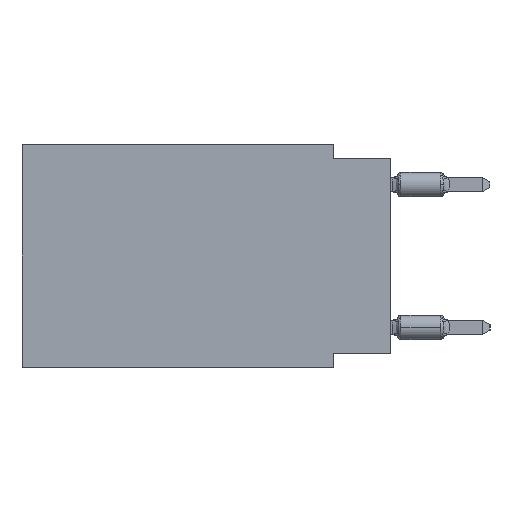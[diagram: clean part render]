
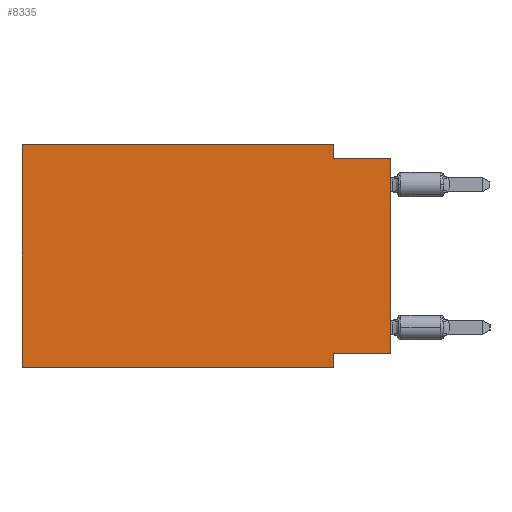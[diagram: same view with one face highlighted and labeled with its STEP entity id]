
A CAD part, left-side view. The second image highlights one B-rep face of the part: STEP entity #8335.
In plain terms, the highlighted planar face has unit normal (-1, 0, 0).
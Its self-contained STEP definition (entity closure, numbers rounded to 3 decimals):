
#430 = CARTESIAN_POINT ( 'NONE',  ( 0., 16.383, 0. ) ) ;
#1123 = LINE ( 'NONE', #44774, #3956 ) ;
#1785 = DIRECTION ( 'NONE',  ( 0., 0., -1. ) ) ;
#2070 = CARTESIAN_POINT ( 'NONE',  ( 0., 2.54, -9.906 ) ) ;
#3323 = LINE ( 'NONE', #20740, #50552 ) ;
#3592 = ORIENTED_EDGE ( 'NONE', *, *, #9408, .F. ) ;
#3956 = VECTOR ( 'NONE', #40205, 1000. ) ;
#3980 = VECTOR ( 'NONE', #14338, 1000. ) ;
#4387 = VECTOR ( 'NONE', #41965, 1000. ) ;
#4584 = EDGE_CURVE ( 'NONE', #22679, #56412, #5011, .T. ) ;
#5011 = LINE ( 'NONE', #22414, #19287 ) ;
#5389 = CARTESIAN_POINT ( 'NONE',  ( 0., 2.54, -9.271 ) ) ;
#5485 = LINE ( 'NONE', #2070, #22809 ) ;
#6275 = EDGE_CURVE ( 'NONE', #49860, #53105, #1123, .T. ) ;
#8335 = ADVANCED_FACE ( 'NONE', ( #8699 ), #44366, .F. ) ;
#8699 = FACE_OUTER_BOUND ( 'NONE', #13908, .T. ) ;
#9408 = EDGE_CURVE ( 'NONE', #38967, #18701, #3323, .T. ) ;
#10695 = CARTESIAN_POINT ( 'NONE',  ( 0., 2.54, 0. ) ) ;
#11708 = ORIENTED_EDGE ( 'NONE', *, *, #31858, .F. ) ;
#13908 = EDGE_LOOP ( 'NONE', ( #37517, #3592, #27225, #41582, #35660, #19641, #11708, #47218 ) ) ;
#14338 = DIRECTION ( 'NONE',  ( 0., 0., 1. ) ) ;
#14681 = CARTESIAN_POINT ( 'NONE',  ( 0., 2.54, -0.635 ) ) ;
#17725 = CARTESIAN_POINT ( 'NONE',  ( 0., 16.383, 0. ) ) ;
#18701 = VERTEX_POINT ( 'NONE', #43627 ) ;
#19269 = DIRECTION ( 'NONE',  ( 0., 0., -1. ) ) ;
#19287 = VECTOR ( 'NONE', #31823, 1000. ) ;
#19641 = ORIENTED_EDGE ( 'NONE', *, *, #21754, .T. ) ;
#20740 = CARTESIAN_POINT ( 'NONE',  ( 0., 0., -0.635 ) ) ;
#20857 = DIRECTION ( 'NONE',  ( 0., -1., 0. ) ) ;
#21614 = CARTESIAN_POINT ( 'NONE',  ( 0., 2.54, -9.906 ) ) ;
#21754 = EDGE_CURVE ( 'NONE', #45782, #35164, #37982, .T. ) ;
#22414 = CARTESIAN_POINT ( 'NONE',  ( 0., 0., -9.271 ) ) ;
#22679 = VERTEX_POINT ( 'NONE', #35497 ) ;
#22809 = VECTOR ( 'NONE', #1785, 1000. ) ;
#22915 = CARTESIAN_POINT ( 'NONE',  ( 0., 16.383, -9.906 ) ) ;
#24866 = CARTESIAN_POINT ( 'NONE',  ( 0., 16.383, -9.906 ) ) ;
#27225 = ORIENTED_EDGE ( 'NONE', *, *, #31450, .F. ) ;
#31192 = VECTOR ( 'NONE', #20857, 1000. ) ;
#31450 = EDGE_CURVE ( 'NONE', #53105, #38967, #44941, .T. ) ;
#31823 = DIRECTION ( 'NONE',  ( 0., 1., 0. ) ) ;
#31858 = EDGE_CURVE ( 'NONE', #56412, #35164, #5485, .T. ) ;
#35164 = VERTEX_POINT ( 'NONE', #21614 ) ;
#35497 = CARTESIAN_POINT ( 'NONE',  ( 0., 0., -9.271 ) ) ;
#35660 = ORIENTED_EDGE ( 'NONE', *, *, #47461, .F. ) ;
#37517 = ORIENTED_EDGE ( 'NONE', *, *, #52344, .T. ) ;
#37863 = AXIS2_PLACEMENT_3D ( 'NONE', #430, #53207, #52084 ) ;
#37982 = LINE ( 'NONE', #24866, #31192 ) ;
#38967 = VERTEX_POINT ( 'NONE', #14681 ) ;
#40205 = DIRECTION ( 'NONE',  ( 0., -1., 0. ) ) ;
#40300 = LINE ( 'NONE', #53420, #3980 ) ;
#41582 = ORIENTED_EDGE ( 'NONE', *, *, #6275, .F. ) ;
#41965 = DIRECTION ( 'NONE',  ( 0., 0., 1. ) ) ;
#43627 = CARTESIAN_POINT ( 'NONE',  ( 0., 0., -0.635 ) ) ;
#44366 = PLANE ( 'NONE',  #37863 ) ;
#44774 = CARTESIAN_POINT ( 'NONE',  ( 0., 16.383, 0. ) ) ;
#44941 = LINE ( 'NONE', #10695, #54694 ) ;
#45680 = LINE ( 'NONE', #54812, #4387 ) ;
#45782 = VERTEX_POINT ( 'NONE', #22915 ) ;
#47218 = ORIENTED_EDGE ( 'NONE', *, *, #4584, .F. ) ;
#47461 = EDGE_CURVE ( 'NONE', #45782, #49860, #45680, .T. ) ;
#49860 = VERTEX_POINT ( 'NONE', #17725 ) ;
#50552 = VECTOR ( 'NONE', #50968, 1000. ) ;
#50968 = DIRECTION ( 'NONE',  ( 0., -1., 0. ) ) ;
#52084 = DIRECTION ( 'NONE',  ( 0., 0., -1. ) ) ;
#52344 = EDGE_CURVE ( 'NONE', #22679, #18701, #40300, .T. ) ;
#53105 = VERTEX_POINT ( 'NONE', #53785 ) ;
#53207 = DIRECTION ( 'NONE',  ( 1., 0., 0. ) ) ;
#53420 = CARTESIAN_POINT ( 'NONE',  ( 0., 0., 0. ) ) ;
#53785 = CARTESIAN_POINT ( 'NONE',  ( 0., 2.54, 0. ) ) ;
#54694 = VECTOR ( 'NONE', #19269, 1000. ) ;
#54812 = CARTESIAN_POINT ( 'NONE',  ( 0., 16.383, 0. ) ) ;
#56412 = VERTEX_POINT ( 'NONE', #5389 ) ;
